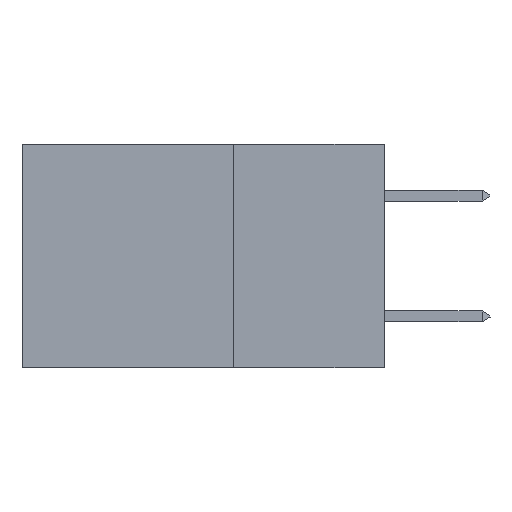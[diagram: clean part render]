
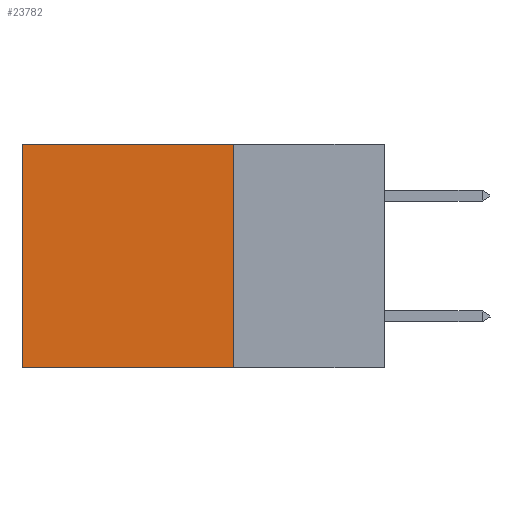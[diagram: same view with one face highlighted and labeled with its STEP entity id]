
A CAD part, left-side view. The second image highlights one B-rep face of the part: STEP entity #23782.
In plain terms, the highlighted planar face has unit normal (-1, 0, 0).
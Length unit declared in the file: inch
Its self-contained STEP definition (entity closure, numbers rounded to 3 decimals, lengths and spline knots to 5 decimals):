
#325 = DIRECTION ( 'NONE',  ( 0., 0., -1. ) ) ;
#543 = VECTOR ( 'NONE', #21638, 39.37008 ) ;
#727 = VERTEX_POINT ( 'NONE', #3968 ) ;
#1006 = CARTESIAN_POINT ( 'NONE',  ( 0.2875, 0.6, 0. ) ) ;
#1466 = ORIENTED_EDGE ( 'NONE', *, *, #9085, .T. ) ;
#1827 = EDGE_CURVE ( 'NONE', #727, #16173, #13039, .T. ) ;
#1856 = AXIS2_PLACEMENT_3D ( 'NONE', #19664, #21719, #325 ) ;
#2235 = VECTOR ( 'NONE', #17557, 39.37008 ) ;
#2598 = VECTOR ( 'NONE', #3775, 39.37008 ) ;
#2834 = CARTESIAN_POINT ( 'NONE',  ( 0.2875, 0.25, -0.37 ) ) ;
#3775 = DIRECTION ( 'NONE',  ( 0., 0., -1. ) ) ;
#3968 = CARTESIAN_POINT ( 'NONE',  ( 0.2875, 0.6, 0. ) ) ;
#6355 = VECTOR ( 'NONE', #11666, 39.37008 ) ;
#6958 = CARTESIAN_POINT ( 'NONE',  ( 0.2875, 0.25, 0. ) ) ;
#7158 = VERTEX_POINT ( 'NONE', #12846 ) ;
#7601 = CARTESIAN_POINT ( 'NONE',  ( 0.2875, 0.25, -0.37 ) ) ;
#9085 = EDGE_CURVE ( 'NONE', #7158, #727, #11045, .T. ) ;
#11045 = LINE ( 'NONE', #29676, #543 ) ;
#11359 = EDGE_LOOP ( 'NONE', ( #22509, #14871, #13032, #1466 ) ) ;
#11666 = DIRECTION ( 'NONE',  ( 0., 0., -1. ) ) ;
#12250 = PLANE ( 'NONE',  #1856 ) ;
#12644 = LINE ( 'NONE', #6958, #6355 ) ;
#12846 = CARTESIAN_POINT ( 'NONE',  ( 0.2875, 0.25, 0. ) ) ;
#13032 = ORIENTED_EDGE ( 'NONE', *, *, #30176, .F. ) ;
#13039 = LINE ( 'NONE', #1006, #2598 ) ;
#14864 = FACE_OUTER_BOUND ( 'NONE', #11359, .T. ) ;
#14871 = ORIENTED_EDGE ( 'NONE', *, *, #23180, .F. ) ;
#16173 = VERTEX_POINT ( 'NONE', #30166 ) ;
#17557 = DIRECTION ( 'NONE',  ( 0., 1., 0. ) ) ;
#19664 = CARTESIAN_POINT ( 'NONE',  ( 0.2875, 0.25, 0. ) ) ;
#21638 = DIRECTION ( 'NONE',  ( 0., 1., 0. ) ) ;
#21719 = DIRECTION ( 'NONE',  ( 1., 0., 0. ) ) ;
#22509 = ORIENTED_EDGE ( 'NONE', *, *, #1827, .T. ) ;
#23180 = EDGE_CURVE ( 'NONE', #26419, #16173, #24755, .T. ) ;
#23782 = ADVANCED_FACE ( 'NONE', ( #14864 ), #12250, .F. ) ;
#24755 = LINE ( 'NONE', #7601, #2235 ) ;
#26419 = VERTEX_POINT ( 'NONE', #2834 ) ;
#29676 = CARTESIAN_POINT ( 'NONE',  ( 0.2875, 0.25, 0. ) ) ;
#30166 = CARTESIAN_POINT ( 'NONE',  ( 0.2875, 0.6, -0.37 ) ) ;
#30176 = EDGE_CURVE ( 'NONE', #7158, #26419, #12644, .T. ) ;
